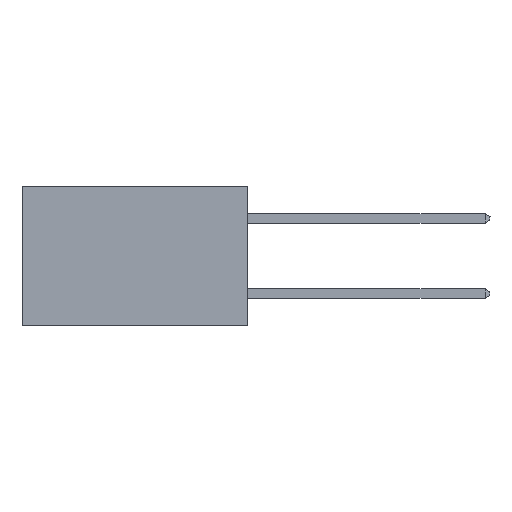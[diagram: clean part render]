
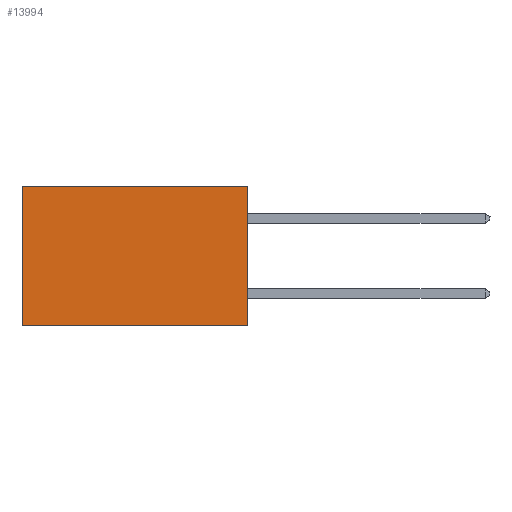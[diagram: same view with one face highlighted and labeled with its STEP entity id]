
A CAD part, left-side view. The second image highlights one B-rep face of the part: STEP entity #13994.
In plain terms, the highlighted planar face has unit normal (-1, 0, 0).
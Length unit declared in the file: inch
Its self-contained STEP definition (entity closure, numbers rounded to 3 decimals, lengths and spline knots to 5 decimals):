
#583 = DIRECTION ( 'NONE',  ( 0., 0., -1. ) ) ;
#1183 = DIRECTION ( 'NONE',  ( 0., 1., 0. ) ) ;
#1263 = CARTESIAN_POINT ( 'NONE',  ( 0.298, 0.6, -0.37 ) ) ;
#1280 = DIRECTION ( 'NONE',  ( 0., 0., -1. ) ) ;
#1336 = EDGE_CURVE ( 'NONE', #18860, #6923, #11220, .T. ) ;
#2094 = VECTOR ( 'NONE', #15112, 39.37008 ) ;
#2606 = CARTESIAN_POINT ( 'NONE',  ( 0.298, 0., 0. ) ) ;
#2780 = AXIS2_PLACEMENT_3D ( 'NONE', #2606, #13799, #4270 ) ;
#2790 = CARTESIAN_POINT ( 'NONE',  ( 0.298, 0., -0.37 ) ) ;
#3556 = ORIENTED_EDGE ( 'NONE', *, *, #19932, .F. ) ;
#4086 = VERTEX_POINT ( 'NONE', #2790 ) ;
#4201 = VERTEX_POINT ( 'NONE', #6450 ) ;
#4270 = DIRECTION ( 'NONE',  ( 0., 0., -1. ) ) ;
#5064 = CARTESIAN_POINT ( 'NONE',  ( 0.298, 0.6, 0. ) ) ;
#5561 = ORIENTED_EDGE ( 'NONE', *, *, #5764, .F. ) ;
#5764 = EDGE_CURVE ( 'NONE', #4086, #6923, #10679, .T. ) ;
#6450 = CARTESIAN_POINT ( 'NONE',  ( 0.298, 0., 0. ) ) ;
#6913 = LINE ( 'NONE', #18300, #2094 ) ;
#6923 = VERTEX_POINT ( 'NONE', #1263 ) ;
#6988 = VECTOR ( 'NONE', #583, 39.37008 ) ;
#8281 = CARTESIAN_POINT ( 'NONE',  ( 0.298, 0., -0.37 ) ) ;
#9840 = VECTOR ( 'NONE', #1280, 39.37008 ) ;
#10679 = LINE ( 'NONE', #8281, #14411 ) ;
#11220 = LINE ( 'NONE', #14408, #6988 ) ;
#12177 = PLANE ( 'NONE',  #2780 ) ;
#13799 = DIRECTION ( 'NONE',  ( 1., 0., 0. ) ) ;
#13801 = EDGE_CURVE ( 'NONE', #4201, #18860, #6913, .T. ) ;
#13994 = ADVANCED_FACE ( 'NONE', ( #15611 ), #12177, .F. ) ;
#14039 = LINE ( 'NONE', #20371, #9840 ) ;
#14408 = CARTESIAN_POINT ( 'NONE',  ( 0.298, 0.6, 0. ) ) ;
#14411 = VECTOR ( 'NONE', #1183, 39.37008 ) ;
#15112 = DIRECTION ( 'NONE',  ( 0., 1., 0. ) ) ;
#15389 = ORIENTED_EDGE ( 'NONE', *, *, #1336, .T. ) ;
#15611 = FACE_OUTER_BOUND ( 'NONE', #18548, .T. ) ;
#16465 = ORIENTED_EDGE ( 'NONE', *, *, #13801, .T. ) ;
#18300 = CARTESIAN_POINT ( 'NONE',  ( 0.298, 0., 0. ) ) ;
#18548 = EDGE_LOOP ( 'NONE', ( #15389, #5561, #3556, #16465 ) ) ;
#18860 = VERTEX_POINT ( 'NONE', #5064 ) ;
#19932 = EDGE_CURVE ( 'NONE', #4201, #4086, #14039, .T. ) ;
#20371 = CARTESIAN_POINT ( 'NONE',  ( 0.298, 0., 0. ) ) ;
